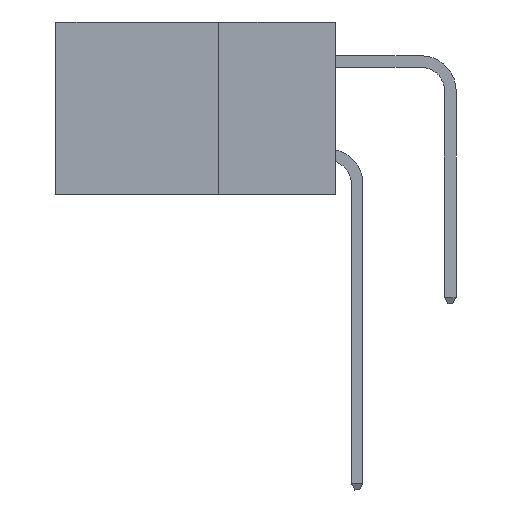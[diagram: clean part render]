
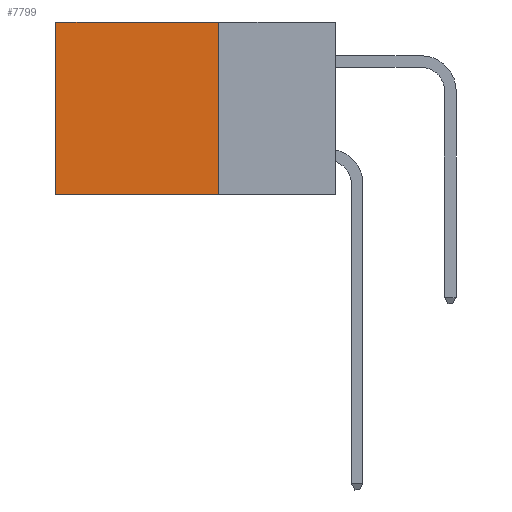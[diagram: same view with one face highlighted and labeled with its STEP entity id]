
A CAD part, left-side view. The second image highlights one B-rep face of the part: STEP entity #7799.
In plain terms, the highlighted planar face has unit normal (-1, 0, 0).
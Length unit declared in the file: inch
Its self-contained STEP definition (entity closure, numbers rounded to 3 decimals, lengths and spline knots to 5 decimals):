
#813 = CARTESIAN_POINT ( 'NONE',  ( 0.2875, 0.25, -0.37 ) ) ;
#1957 = VERTEX_POINT ( 'NONE', #813 ) ;
#2036 = CARTESIAN_POINT ( 'NONE',  ( 0.2875, 0.6, -0.37 ) ) ;
#2322 = CARTESIAN_POINT ( 'NONE',  ( 0.2875, 0.25, 0. ) ) ;
#2699 = AXIS2_PLACEMENT_3D ( 'NONE', #2322, #6409, #10841 ) ;
#2704 = DIRECTION ( 'NONE',  ( 0., 0., -1. ) ) ;
#3977 = ORIENTED_EDGE ( 'NONE', *, *, #11230, .F. ) ;
#4690 = EDGE_CURVE ( 'NONE', #14726, #8217, #16133, .T. ) ;
#5102 = VECTOR ( 'NONE', #10878, 39.37008 ) ;
#5400 = VECTOR ( 'NONE', #10403, 39.37008 ) ;
#5450 = VECTOR ( 'NONE', #2704, 39.37008 ) ;
#5477 = CARTESIAN_POINT ( 'NONE',  ( 0.2875, 0.25, 0. ) ) ;
#6409 = DIRECTION ( 'NONE',  ( 1., 0., 0. ) ) ;
#6921 = CARTESIAN_POINT ( 'NONE',  ( 0.2875, 0.25, 0. ) ) ;
#7044 = CARTESIAN_POINT ( 'NONE',  ( 0.2875, 0.25, -0.37 ) ) ;
#7799 = ADVANCED_FACE ( 'NONE', ( #12029 ), #8073, .F. ) ;
#8073 = PLANE ( 'NONE',  #2699 ) ;
#8217 = VERTEX_POINT ( 'NONE', #11751 ) ;
#9287 = ORIENTED_EDGE ( 'NONE', *, *, #4690, .T. ) ;
#10403 = DIRECTION ( 'NONE',  ( 0., 0., -1. ) ) ;
#10841 = DIRECTION ( 'NONE',  ( 0., 0., -1. ) ) ;
#10878 = DIRECTION ( 'NONE',  ( 0., 1., 0. ) ) ;
#11230 = EDGE_CURVE ( 'NONE', #14726, #1957, #15792, .T. ) ;
#11604 = EDGE_LOOP ( 'NONE', ( #14261, #11618, #3977, #9287 ) ) ;
#11618 = ORIENTED_EDGE ( 'NONE', *, *, #15573, .F. ) ;
#11751 = CARTESIAN_POINT ( 'NONE',  ( 0.2875, 0.6, 0. ) ) ;
#12029 = FACE_OUTER_BOUND ( 'NONE', #11604, .T. ) ;
#12760 = DIRECTION ( 'NONE',  ( 0., 1., 0. ) ) ;
#12952 = EDGE_CURVE ( 'NONE', #8217, #15157, #13126, .T. ) ;
#13122 = CARTESIAN_POINT ( 'NONE',  ( 0.2875, 0.6, 0. ) ) ;
#13126 = LINE ( 'NONE', #13122, #5400 ) ;
#13227 = CARTESIAN_POINT ( 'NONE',  ( 0.2875, 0.25, 0. ) ) ;
#13375 = VECTOR ( 'NONE', #12760, 39.37008 ) ;
#14261 = ORIENTED_EDGE ( 'NONE', *, *, #12952, .T. ) ;
#14726 = VERTEX_POINT ( 'NONE', #13227 ) ;
#15157 = VERTEX_POINT ( 'NONE', #2036 ) ;
#15558 = LINE ( 'NONE', #7044, #13375 ) ;
#15573 = EDGE_CURVE ( 'NONE', #1957, #15157, #15558, .T. ) ;
#15792 = LINE ( 'NONE', #6921, #5450 ) ;
#16133 = LINE ( 'NONE', #5477, #5102 ) ;
